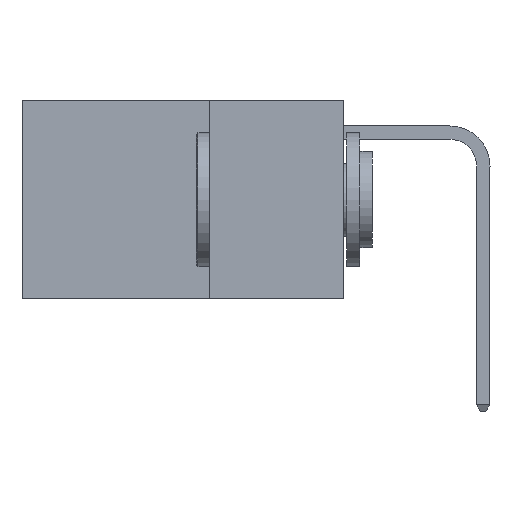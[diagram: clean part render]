
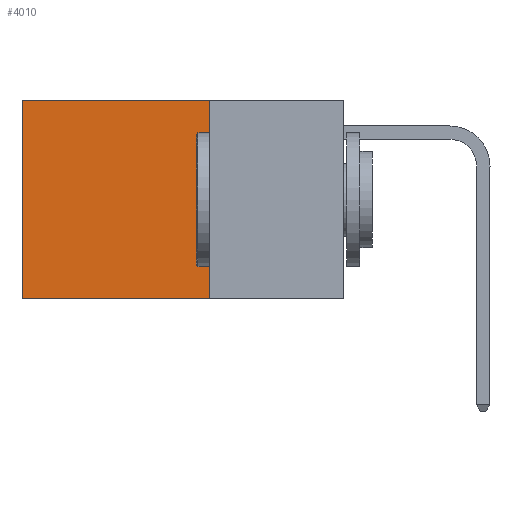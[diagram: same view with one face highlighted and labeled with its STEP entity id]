
A CAD part, left-side view. The second image highlights one B-rep face of the part: STEP entity #4010.
In plain terms, the highlighted planar face has unit normal (-1, 0, 0).
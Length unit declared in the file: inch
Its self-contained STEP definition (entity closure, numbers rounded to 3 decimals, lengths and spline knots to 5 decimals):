
#138 = VERTEX_POINT ( 'NONE', #5012 ) ;
#232 = CARTESIAN_POINT ( 'NONE',  ( 0.2625, 0.25, 0. ) ) ;
#777 = AXIS2_PLACEMENT_3D ( 'NONE', #12548, #9369, #20623 ) ;
#1257 = CARTESIAN_POINT ( 'NONE',  ( 0.2625, 0.6, 0. ) ) ;
#1895 = DIRECTION ( 'NONE',  ( 0., 0., -1. ) ) ;
#2341 = EDGE_CURVE ( 'NONE', #12355, #138, #19479, .T. ) ;
#3642 = LINE ( 'NONE', #232, #6924 ) ;
#4010 = ADVANCED_FACE ( 'NONE', ( #10647 ), #19008, .F. ) ;
#4612 = LINE ( 'NONE', #5932, #16999 ) ;
#5012 = CARTESIAN_POINT ( 'NONE',  ( 0.2625, 0.6, -0.37 ) ) ;
#5037 = ORIENTED_EDGE ( 'NONE', *, *, #7299, .T. ) ;
#5222 = EDGE_LOOP ( 'NONE', ( #10847, #12167, #7816, #5037 ) ) ;
#5705 = LINE ( 'NONE', #12874, #9531 ) ;
#5932 = CARTESIAN_POINT ( 'NONE',  ( 0.2625, 0.6, 0. ) ) ;
#6924 = VECTOR ( 'NONE', #1895, 39.37008 ) ;
#7299 = EDGE_CURVE ( 'NONE', #14642, #12438, #5705, .T. ) ;
#7816 = ORIENTED_EDGE ( 'NONE', *, *, #13940, .F. ) ;
#8048 = DIRECTION ( 'NONE',  ( 0., 1., 0. ) ) ;
#9369 = DIRECTION ( 'NONE',  ( 1., 0., 0. ) ) ;
#9531 = VECTOR ( 'NONE', #8048, 39.37008 ) ;
#9754 = EDGE_CURVE ( 'NONE', #12438, #138, #4612, .T. ) ;
#10422 = DIRECTION ( 'NONE',  ( 0., 1., 0. ) ) ;
#10647 = FACE_OUTER_BOUND ( 'NONE', #5222, .T. ) ;
#10811 = DIRECTION ( 'NONE',  ( 0., 0., -1. ) ) ;
#10847 = ORIENTED_EDGE ( 'NONE', *, *, #9754, .T. ) ;
#11849 = CARTESIAN_POINT ( 'NONE',  ( 0.2625, 0.25, 0. ) ) ;
#12167 = ORIENTED_EDGE ( 'NONE', *, *, #2341, .F. ) ;
#12355 = VERTEX_POINT ( 'NONE', #18770 ) ;
#12438 = VERTEX_POINT ( 'NONE', #1257 ) ;
#12548 = CARTESIAN_POINT ( 'NONE',  ( 0.2625, 0.25, 0. ) ) ;
#12620 = CARTESIAN_POINT ( 'NONE',  ( 0.2625, 0.25, -0.37 ) ) ;
#12874 = CARTESIAN_POINT ( 'NONE',  ( 0.2625, 0.25, 0. ) ) ;
#13940 = EDGE_CURVE ( 'NONE', #14642, #12355, #3642, .T. ) ;
#14642 = VERTEX_POINT ( 'NONE', #11849 ) ;
#16702 = VECTOR ( 'NONE', #10422, 39.37008 ) ;
#16999 = VECTOR ( 'NONE', #10811, 39.37008 ) ;
#18770 = CARTESIAN_POINT ( 'NONE',  ( 0.2625, 0.25, -0.37 ) ) ;
#19008 = PLANE ( 'NONE',  #777 ) ;
#19479 = LINE ( 'NONE', #12620, #16702 ) ;
#20623 = DIRECTION ( 'NONE',  ( 0., 0., -1. ) ) ;
